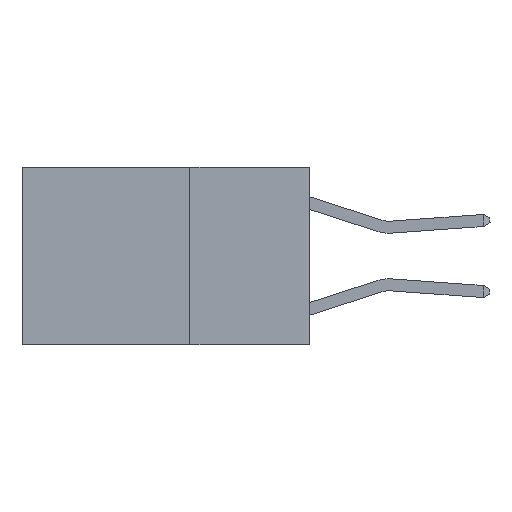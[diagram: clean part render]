
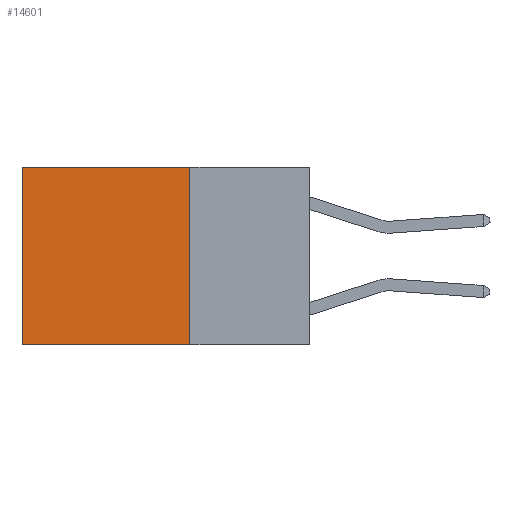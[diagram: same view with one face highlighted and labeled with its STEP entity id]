
A CAD part, left-side view. The second image highlights one B-rep face of the part: STEP entity #14601.
In plain terms, the highlighted planar face has unit normal (-1, 0, 0).
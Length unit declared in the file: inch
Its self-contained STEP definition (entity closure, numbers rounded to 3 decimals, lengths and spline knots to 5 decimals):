
#446 = VECTOR ( 'NONE', #17331, 39.37008 ) ;
#509 = CARTESIAN_POINT ( 'NONE',  ( 0.2625, 0.6, -0.37 ) ) ;
#820 = DIRECTION ( 'NONE',  ( 0., 0., -1. ) ) ;
#957 = ORIENTED_EDGE ( 'NONE', *, *, #4812, .F. ) ;
#2121 = CARTESIAN_POINT ( 'NONE',  ( 0.2625, 0.25, 0. ) ) ;
#2303 = CARTESIAN_POINT ( 'NONE',  ( 0.2625, 0.6, 0. ) ) ;
#3259 = EDGE_CURVE ( 'NONE', #5913, #8561, #11449, .T. ) ;
#4401 = CARTESIAN_POINT ( 'NONE',  ( 0.2625, 0.25, -0.37 ) ) ;
#4812 = EDGE_CURVE ( 'NONE', #16040, #6636, #11414, .T. ) ;
#5489 = CARTESIAN_POINT ( 'NONE',  ( 0.2625, 0.25, 0. ) ) ;
#5678 = DIRECTION ( 'NONE',  ( 0., 0., -1. ) ) ;
#5913 = VERTEX_POINT ( 'NONE', #2121 ) ;
#6208 = EDGE_LOOP ( 'NONE', ( #11807, #957, #15180, #15999 ) ) ;
#6211 = LINE ( 'NONE', #12346, #15823 ) ;
#6220 = CARTESIAN_POINT ( 'NONE',  ( 0.2625, 0.25, -0.37 ) ) ;
#6636 = VERTEX_POINT ( 'NONE', #509 ) ;
#8006 = CARTESIAN_POINT ( 'NONE',  ( 0.2625, 0.6, 0. ) ) ;
#8561 = VERTEX_POINT ( 'NONE', #2303 ) ;
#10390 = DIRECTION ( 'NONE',  ( 0., 1., 0. ) ) ;
#11125 = DIRECTION ( 'NONE',  ( 1., 0., 0. ) ) ;
#11414 = LINE ( 'NONE', #4401, #13699 ) ;
#11449 = LINE ( 'NONE', #17068, #446 ) ;
#11461 = EDGE_CURVE ( 'NONE', #8561, #6636, #13546, .T. ) ;
#11807 = ORIENTED_EDGE ( 'NONE', *, *, #11461, .T. ) ;
#12346 = CARTESIAN_POINT ( 'NONE',  ( 0.2625, 0.25, 0. ) ) ;
#13546 = LINE ( 'NONE', #8006, #13548 ) ;
#13548 = VECTOR ( 'NONE', #820, 39.37008 ) ;
#13699 = VECTOR ( 'NONE', #10390, 39.37008 ) ;
#13970 = PLANE ( 'NONE',  #13972 ) ;
#13972 = AXIS2_PLACEMENT_3D ( 'NONE', #5489, #11125, #5678 ) ;
#14601 = ADVANCED_FACE ( 'NONE', ( #16919 ), #13970, .F. ) ;
#15102 = DIRECTION ( 'NONE',  ( 0., 0., -1. ) ) ;
#15180 = ORIENTED_EDGE ( 'NONE', *, *, #17555, .F. ) ;
#15823 = VECTOR ( 'NONE', #15102, 39.37008 ) ;
#15999 = ORIENTED_EDGE ( 'NONE', *, *, #3259, .T. ) ;
#16040 = VERTEX_POINT ( 'NONE', #6220 ) ;
#16919 = FACE_OUTER_BOUND ( 'NONE', #6208, .T. ) ;
#17068 = CARTESIAN_POINT ( 'NONE',  ( 0.2625, 0.25, 0. ) ) ;
#17331 = DIRECTION ( 'NONE',  ( 0., 1., 0. ) ) ;
#17555 = EDGE_CURVE ( 'NONE', #5913, #16040, #6211, .T. ) ;
